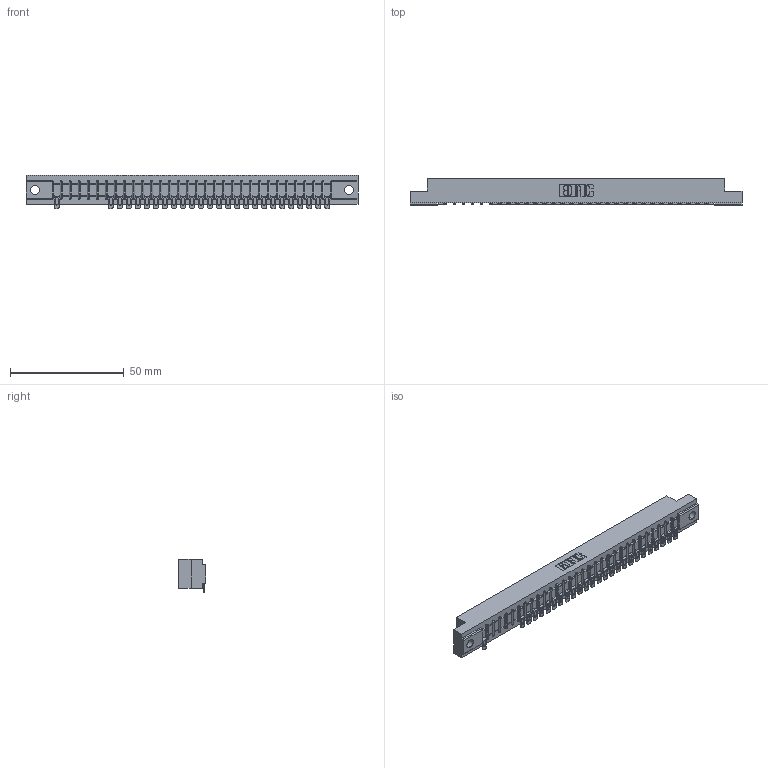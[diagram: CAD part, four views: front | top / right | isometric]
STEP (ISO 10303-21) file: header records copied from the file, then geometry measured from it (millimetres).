
FILE_DESCRIPTION (( 'STEP AP203' ), '1' );
FILE_NAME ('357-031-554-104.STEP', '2018-08-09T22:52:20', ( '' ), ( '' ), 'SwSTEP 2.0', 'SolidWorks 2016', '' );
FILE_SCHEMA (( 'CONFIG_CONTROL_DESIGN' ));
Length unit declared in the file: inch
Products named in the file (3): 307 Part_.156 Dia Mounting Holes; 307-290-002_554; 357-031-554-104
Assembly tree (27 placements, depth 2):
  357-031-554-104
    307 Part_.156 Dia Mounting Holes
    307-290-002_554  x26
Bounding box: 145.85 x 12.01 x 14.52 mm (x, y, z)
Volume: 15284.2 mm3; surface area: 17986.1 mm2
Topology: 27 solids, 27 shells, 2370 faces, 7257 edges, 4750 vertices
Faces by surface type: plane 1340, cylinder 966, sphere 64
Entity records: 29155 total; most frequent: CARTESIAN_POINT 4943, ORIENTED_EDGE 4936, DIRECTION 4800, EDGE_CURVE 2468, LINE 1886, VECTOR 1886, VERTEX_POINT 1600, AXIS2_PLACEMENT_3D 1457
